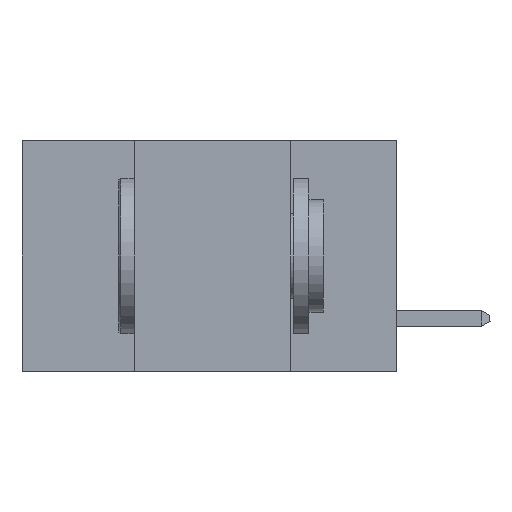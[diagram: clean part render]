
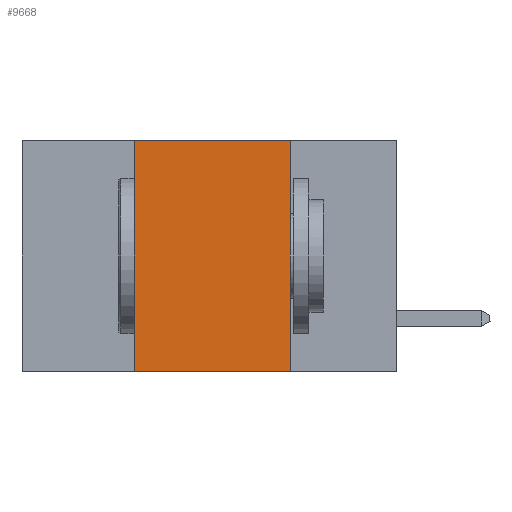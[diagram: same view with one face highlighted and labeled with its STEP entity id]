
A CAD part, left-side view. The second image highlights one B-rep face of the part: STEP entity #9668.
In plain terms, the highlighted planar face has unit normal (-1, 0, 0).
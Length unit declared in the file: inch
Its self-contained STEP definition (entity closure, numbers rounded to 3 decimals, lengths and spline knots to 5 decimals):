
#718 = VECTOR ( 'NONE', #10833, 39.37008 ) ;
#1647 = EDGE_CURVE ( 'NONE', #9338, #5454, #6163, .T. ) ;
#1730 = PLANE ( 'NONE',  #3612 ) ;
#1806 = VECTOR ( 'NONE', #6474, 39.37008 ) ;
#2202 = EDGE_CURVE ( 'NONE', #11921, #3826, #4114, .T. ) ;
#2238 = CARTESIAN_POINT ( 'NONE',  ( 0., 0.17, 0. ) ) ;
#2641 = CARTESIAN_POINT ( 'NONE',  ( 0., 0.42, -0.37 ) ) ;
#2959 = CARTESIAN_POINT ( 'NONE',  ( 0., 0.6, 0. ) ) ;
#3612 = AXIS2_PLACEMENT_3D ( 'NONE', #2959, #4256, #12447 ) ;
#3826 = VERTEX_POINT ( 'NONE', #4569 ) ;
#4114 = LINE ( 'NONE', #12872, #718 ) ;
#4256 = DIRECTION ( 'NONE',  ( 1., 0., 0. ) ) ;
#4569 = CARTESIAN_POINT ( 'NONE',  ( 0., 0.17, -0.37 ) ) ;
#5454 = VERTEX_POINT ( 'NONE', #2238 ) ;
#6154 = FACE_OUTER_BOUND ( 'NONE', #14304, .T. ) ;
#6163 = LINE ( 'NONE', #13352, #11293 ) ;
#6239 = ORIENTED_EDGE ( 'NONE', *, *, #12826, .F. ) ;
#6474 = DIRECTION ( 'NONE',  ( 0., 0., -1. ) ) ;
#7730 = ORIENTED_EDGE ( 'NONE', *, *, #2202, .T. ) ;
#9338 = VERTEX_POINT ( 'NONE', #9488 ) ;
#9488 = CARTESIAN_POINT ( 'NONE',  ( 0., 0.42, 0. ) ) ;
#9668 = ADVANCED_FACE ( 'NONE', ( #6154 ), #1730, .F. ) ;
#10012 = CARTESIAN_POINT ( 'NONE',  ( 0., 0.17, 0. ) ) ;
#10282 = CARTESIAN_POINT ( 'NONE',  ( 0., 0.42, 0. ) ) ;
#10522 = EDGE_CURVE ( 'NONE', #5454, #3826, #11352, .T. ) ;
#10638 = ORIENTED_EDGE ( 'NONE', *, *, #1647, .F. ) ;
#10733 = LINE ( 'NONE', #10282, #14124 ) ;
#10833 = DIRECTION ( 'NONE',  ( 0., -1., 0. ) ) ;
#11293 = VECTOR ( 'NONE', #14516, 39.37008 ) ;
#11352 = LINE ( 'NONE', #10012, #1806 ) ;
#11921 = VERTEX_POINT ( 'NONE', #2641 ) ;
#12447 = DIRECTION ( 'NONE',  ( 0., 0., -1. ) ) ;
#12591 = ORIENTED_EDGE ( 'NONE', *, *, #10522, .F. ) ;
#12826 = EDGE_CURVE ( 'NONE', #11921, #9338, #10733, .T. ) ;
#12872 = CARTESIAN_POINT ( 'NONE',  ( 0., 0.6, -0.37 ) ) ;
#13352 = CARTESIAN_POINT ( 'NONE',  ( 0., 0.6, 0. ) ) ;
#14124 = VECTOR ( 'NONE', #14821, 39.37008 ) ;
#14304 = EDGE_LOOP ( 'NONE', ( #12591, #10638, #6239, #7730 ) ) ;
#14516 = DIRECTION ( 'NONE',  ( 0., -1., 0. ) ) ;
#14821 = DIRECTION ( 'NONE',  ( 0., 0., 1. ) ) ;
